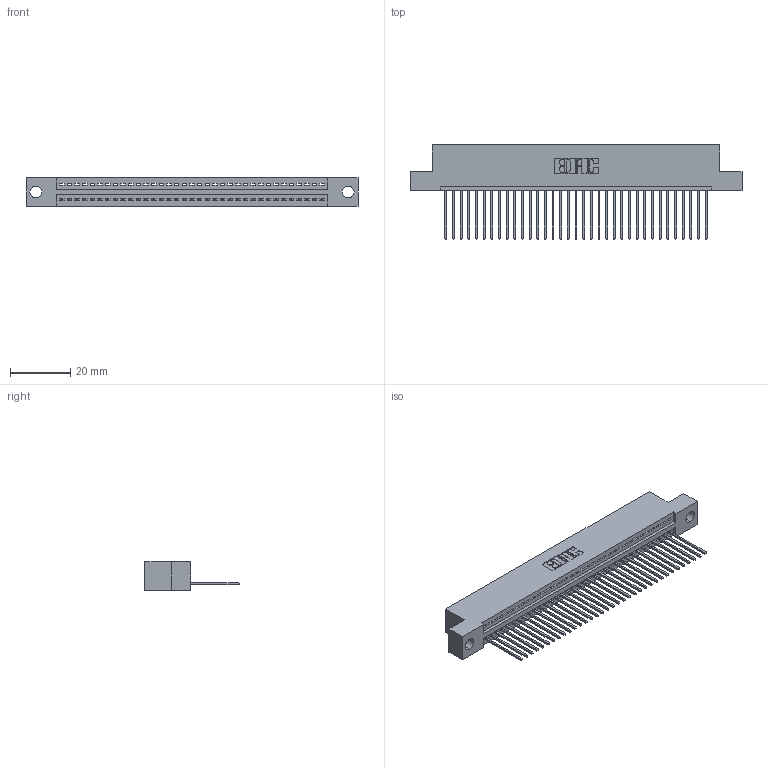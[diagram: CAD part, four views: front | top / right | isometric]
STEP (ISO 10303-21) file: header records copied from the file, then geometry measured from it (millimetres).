
FILE_DESCRIPTION (( 'STEP AP203' ), '1' );
FILE_NAME ('395-035-542-104.STEP', '2021-05-31T14:52:32', ( '' ), ( '' ), 'SwSTEP 2.0', 'SolidWorks 2020', '' );
FILE_SCHEMA (( 'CONFIG_CONTROL_DESIGN' ));
Length unit declared in the file: inch
Products named in the file (3): 395-035-542-104; 345-292-001_345-293-142; 345 Part_Flush Mounting Lugs - 0.156 Dia-TI
Assembly tree (36 placements, depth 2):
  395-035-542-104
    345 Part_Flush Mounting Lugs - 0.156 Dia-TI
    345-292-001_345-293-142  x35
Bounding box: 110.11 x 31.29 x 9.4 mm (x, y, z)
Volume: 10372.8 mm3; surface area: 14024.4 mm2
Topology: 36 solids, 36 shells, 2170 faces, 6537 edges, 4310 vertices
Faces by surface type: plane 1494, cylinder 676
Entity records: 27721 total; most frequent: CARTESIAN_POINT 4811, ORIENTED_EDGE 4778, DIRECTION 4211, EDGE_CURVE 2389, LINE 2117, VECTOR 2117, VERTEX_POINT 1590, AXIS2_PLACEMENT_3D 1047
